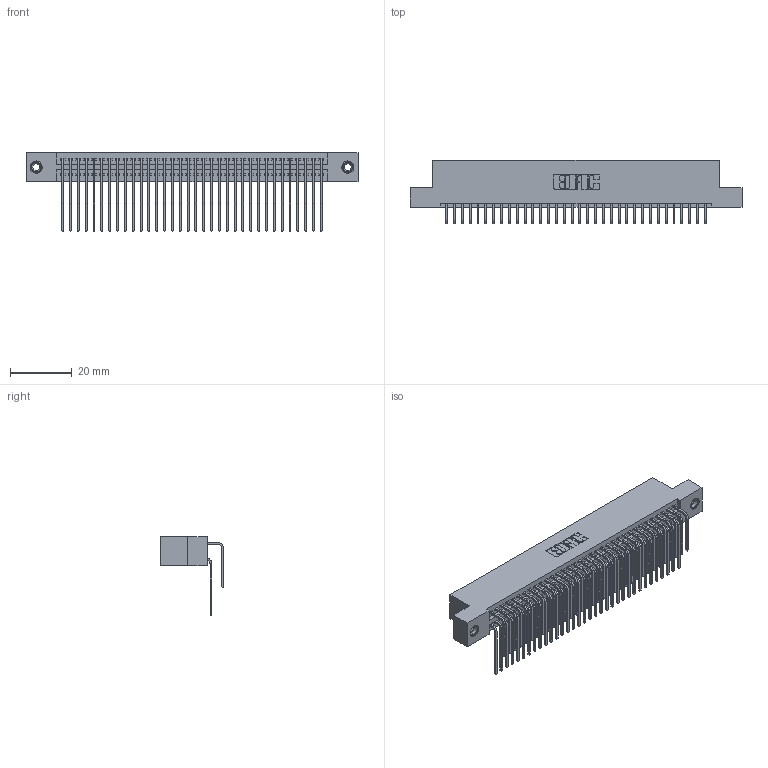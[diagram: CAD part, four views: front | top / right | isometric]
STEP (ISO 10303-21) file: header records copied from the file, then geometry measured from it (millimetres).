
FILE_DESCRIPTION (( 'STEP AP203' ), '1' );
FILE_NAME ('395-068-559-208.STEP', '2019-10-23T23:46:59', ( '' ), ( '' ), 'SwSTEP 2.0', 'SolidWorks 2016', '' );
FILE_SCHEMA (( 'CONFIG_CONTROL_DESIGN' ));
Length unit declared in the file: inch
Products named in the file (5): 345 Part_Flush Mounting Lugs - 0.156 Dia-TI; 345-292-001_558 559 Tail - 1; 345-292-001_559 Tail - 2; 345-250-001_345-250-003-102; 395-068-559-208
Assembly tree (71 placements, depth 2):
  395-068-559-208
    345 Part_Flush Mounting Lugs - 0.156 Dia-TI
    345-292-001_558 559 Tail - 1  x34
    345-292-001_559 Tail - 2  x34
    345-250-001_345-250-003-102  x2
Bounding box: 107.57 x 20.56 x 25.53 mm (x, y, z)
Volume: 10760.9 mm3; surface area: 17609.4 mm2
Topology: 71 solids, 71 shells, 3722 faces, 11017 edges, 7246 vertices
Faces by surface type: plane 2492, cylinder 1214, cone 12, torus 4
Entity records: 30592 total; most frequent: CARTESIAN_POINT 5162, ORIENTED_EDGE 5038, DIRECTION 4561, EDGE_CURVE 2519, LINE 2191, VECTOR 2191, VERTEX_POINT 1672, AXIS2_PLACEMENT_3D 1185
